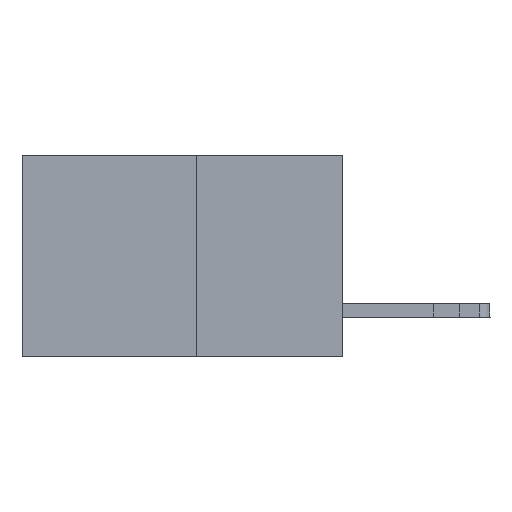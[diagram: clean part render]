
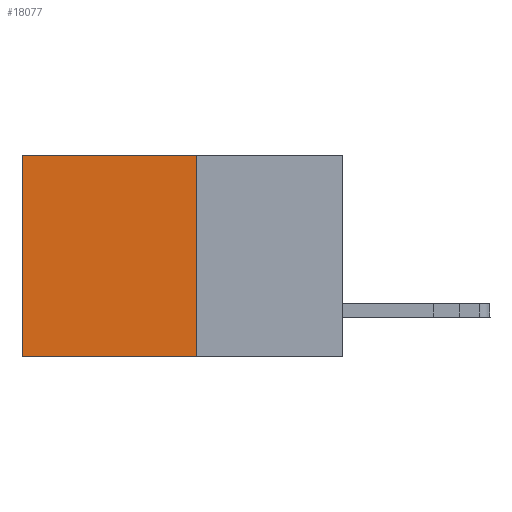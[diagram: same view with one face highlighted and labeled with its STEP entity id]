
A CAD part, left-side view. The second image highlights one B-rep face of the part: STEP entity #18077.
In plain terms, the highlighted planar face has unit normal (-1, 0, 0).
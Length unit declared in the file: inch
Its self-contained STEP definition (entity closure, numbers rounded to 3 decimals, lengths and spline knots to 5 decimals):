
#295 = LINE ( 'NONE', #13579, #4529 ) ;
#1671 = VECTOR ( 'NONE', #7290, 39.37008 ) ;
#1820 = EDGE_CURVE ( 'NONE', #14811, #21090, #10112, .T. ) ;
#2659 = CARTESIAN_POINT ( 'NONE',  ( 0.277, 0.59, -0.37 ) ) ;
#3266 = EDGE_CURVE ( 'NONE', #9925, #14811, #15926, .T. ) ;
#3738 = LINE ( 'NONE', #6204, #17483 ) ;
#4399 = VERTEX_POINT ( 'NONE', #8096 ) ;
#4529 = VECTOR ( 'NONE', #4661, 39.37008 ) ;
#4627 = CARTESIAN_POINT ( 'NONE',  ( 0.277, 0.27, -0.37 ) ) ;
#4661 = DIRECTION ( 'NONE',  ( 0., 1., 0. ) ) ;
#4818 = CARTESIAN_POINT ( 'NONE',  ( 0.277, 0.59, 0. ) ) ;
#6204 = CARTESIAN_POINT ( 'NONE',  ( 0.277, 0.27, -0.37 ) ) ;
#6337 = ORIENTED_EDGE ( 'NONE', *, *, #3266, .T. ) ;
#6415 = DIRECTION ( 'NONE',  ( 0., 0., -1. ) ) ;
#6795 = CARTESIAN_POINT ( 'NONE',  ( 0.277, 0.59, -0.37 ) ) ;
#7290 = DIRECTION ( 'NONE',  ( 0., 0., -1. ) ) ;
#8096 = CARTESIAN_POINT ( 'NONE',  ( 0.277, 0.27, -0.37 ) ) ;
#9925 = VERTEX_POINT ( 'NONE', #15310 ) ;
#10112 = LINE ( 'NONE', #6795, #1671 ) ;
#11171 = VECTOR ( 'NONE', #19662, 39.37008 ) ;
#13579 = CARTESIAN_POINT ( 'NONE',  ( 0.277, 0.27, -0.37 ) ) ;
#14811 = VERTEX_POINT ( 'NONE', #4818 ) ;
#15310 = CARTESIAN_POINT ( 'NONE',  ( 0.277, 0.27, 0. ) ) ;
#15926 = LINE ( 'NONE', #19783, #11171 ) ;
#16003 = ORIENTED_EDGE ( 'NONE', *, *, #16637, .F. ) ;
#16637 = EDGE_CURVE ( 'NONE', #4399, #21090, #295, .T. ) ;
#16719 = EDGE_LOOP ( 'NONE', ( #20853, #16003, #17466, #6337 ) ) ;
#16958 = DIRECTION ( 'NONE',  ( 0., 0., -1. ) ) ;
#17169 = DIRECTION ( 'NONE',  ( 1., 0., 0. ) ) ;
#17466 = ORIENTED_EDGE ( 'NONE', *, *, #23246, .F. ) ;
#17483 = VECTOR ( 'NONE', #16958, 39.37008 ) ;
#17885 = AXIS2_PLACEMENT_3D ( 'NONE', #4627, #17169, #6415 ) ;
#18001 = FACE_OUTER_BOUND ( 'NONE', #16719, .T. ) ;
#18077 = ADVANCED_FACE ( 'NONE', ( #18001 ), #20738, .F. ) ;
#19662 = DIRECTION ( 'NONE',  ( 0., 1., 0. ) ) ;
#19783 = CARTESIAN_POINT ( 'NONE',  ( 0.277, 0.27, 0. ) ) ;
#20738 = PLANE ( 'NONE',  #17885 ) ;
#20853 = ORIENTED_EDGE ( 'NONE', *, *, #1820, .T. ) ;
#21090 = VERTEX_POINT ( 'NONE', #2659 ) ;
#23246 = EDGE_CURVE ( 'NONE', #9925, #4399, #3738, .T. ) ;
